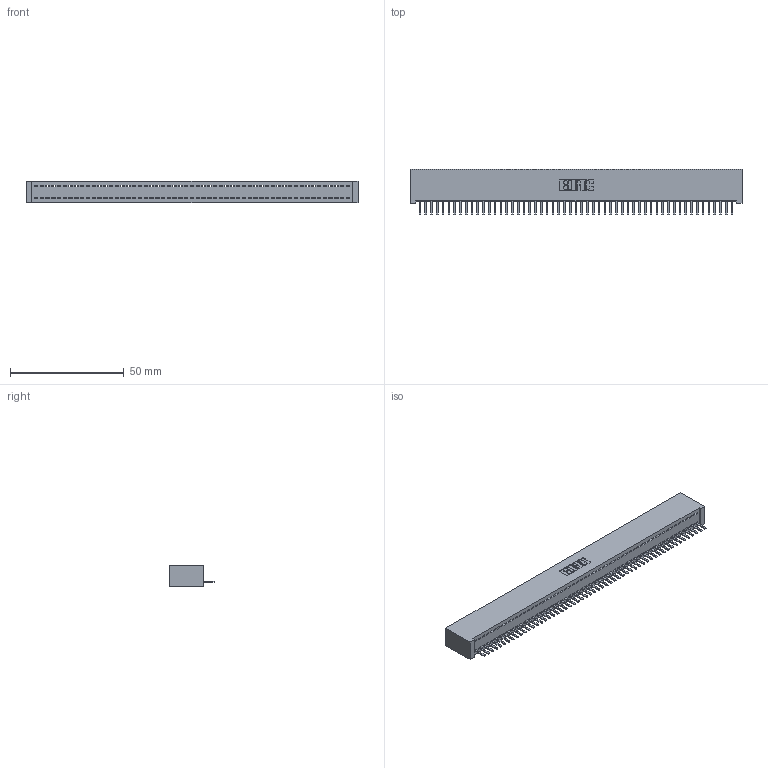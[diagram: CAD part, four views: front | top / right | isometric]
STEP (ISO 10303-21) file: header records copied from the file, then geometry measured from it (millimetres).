
FILE_DESCRIPTION (( 'STEP AP203' ), '1' );
FILE_NAME ('392-055-520-101.STEP', '2019-10-08T14:17:21', ( '' ), ( '' ), 'SwSTEP 2.0', 'SolidWorks 2016', '' );
FILE_SCHEMA (( 'CONFIG_CONTROL_DESIGN' ));
Length unit declared in the file: inch
Products named in the file (3): 342 Part_Lugless; 345-292-001_345-293-120; 392-055-520-101
Assembly tree (56 placements, depth 2):
  392-055-520-101
    342 Part_Lugless
    345-292-001_345-293-120  x55
Bounding box: 145.95 x 20.02 x 9.4 mm (x, y, z)
Volume: 13095.4 mm3; surface area: 19290 mm2
Topology: 56 solids, 56 shells, 3512 faces, 10395 edges, 6782 vertices
Faces by surface type: plane 2482, cylinder 1030
Entity records: 31647 total; most frequent: CARTESIAN_POINT 5475, ORIENTED_EDGE 5454, DIRECTION 4573, EDGE_CURVE 2727, VECTOR 2603, LINE 2603, VERTEX_POINT 1814, AXIS2_PLACEMENT_3D 985
